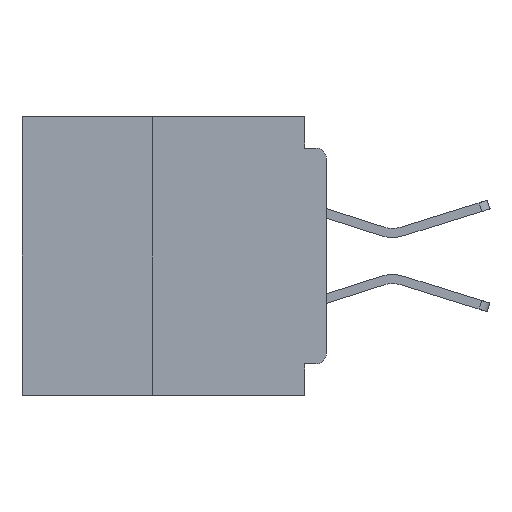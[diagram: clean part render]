
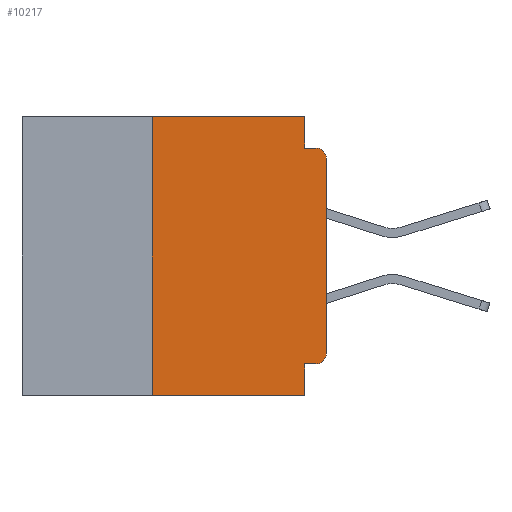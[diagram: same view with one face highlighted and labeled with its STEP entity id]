
A CAD part, left-side view. The second image highlights one B-rep face of the part: STEP entity #10217.
In plain terms, the highlighted planar face has unit normal (-1, 0, 0).
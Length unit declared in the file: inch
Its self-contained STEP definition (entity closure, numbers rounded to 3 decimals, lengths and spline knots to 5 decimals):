
#498 = CIRCLE ( 'NONE', #4912, 0.015 ) ;
#884 = EDGE_CURVE ( 'NONE', #46273, #10649, #34184, .T. ) ;
#911 = ORIENTED_EDGE ( 'NONE', *, *, #20412, .F. ) ;
#1662 = AXIS2_PLACEMENT_3D ( 'NONE', #39921, #15898, #43941 ) ;
#2048 = ORIENTED_EDGE ( 'NONE', *, *, #2463, .F. ) ;
#2142 = VERTEX_POINT ( 'NONE', #7467 ) ;
#2463 = EDGE_CURVE ( 'NONE', #22244, #46273, #28399, .T. ) ;
#3610 = EDGE_CURVE ( 'NONE', #47137, #48964, #48916, .T. ) ;
#3643 = ORIENTED_EDGE ( 'NONE', *, *, #884, .F. ) ;
#4256 = CARTESIAN_POINT ( 'NONE',  ( 0., 0., -0.045 ) ) ;
#4887 = DIRECTION ( 'NONE',  ( 0., -1., 0. ) ) ;
#4912 = AXIS2_PLACEMENT_3D ( 'NONE', #46731, #22721, #50726 ) ;
#5060 = CARTESIAN_POINT ( 'NONE',  ( 0., 0.031, 0. ) ) ;
#5087 = VECTOR ( 'NONE', #30559, 39.37008 ) ;
#5293 = CARTESIAN_POINT ( 'NONE',  ( 0., 0.031, 0. ) ) ;
#6750 = LINE ( 'NONE', #5293, #48163 ) ;
#7467 = CARTESIAN_POINT ( 'NONE',  ( 0., 0.031, -0.4 ) ) ;
#7532 = DIRECTION ( 'NONE',  ( 0., -1., 0. ) ) ;
#7819 = EDGE_CURVE ( 'NONE', #34280, #49689, #32407, .T. ) ;
#7886 = LINE ( 'NONE', #27596, #49278 ) ;
#9709 = DIRECTION ( 'NONE',  ( 0., 1., 0. ) ) ;
#10217 = ADVANCED_FACE ( 'NONE', ( #42195 ), #37605, .F. ) ;
#10649 = VERTEX_POINT ( 'NONE', #5060 ) ;
#10963 = EDGE_CURVE ( 'NONE', #33934, #2142, #45840, .T. ) ;
#11581 = CARTESIAN_POINT ( 'NONE',  ( 0., 0.25, -0.4 ) ) ;
#12179 = EDGE_LOOP ( 'NONE', ( #19804, #41175, #29316, #911, #3643, #2048, #46220, #25577, #29150, #15130 ) ) ;
#13607 = CARTESIAN_POINT ( 'NONE',  ( 0., 0.437, 0. ) ) ;
#13800 = CARTESIAN_POINT ( 'NONE',  ( 0., 0.25, 0. ) ) ;
#14956 = CARTESIAN_POINT ( 'NONE',  ( 0., 0.015, -0.355 ) ) ;
#15130 = ORIENTED_EDGE ( 'NONE', *, *, #7819, .T. ) ;
#15285 = DIRECTION ( 'NONE',  ( 0., 0., -1. ) ) ;
#15851 = LINE ( 'NONE', #50484, #5087 ) ;
#15898 = DIRECTION ( 'NONE',  ( -1., 0., 0. ) ) ;
#17641 = DIRECTION ( 'NONE',  ( 0., 0., -1. ) ) ;
#17723 = VECTOR ( 'NONE', #36551, 39.37008 ) ;
#19588 = VERTEX_POINT ( 'NONE', #20359 ) ;
#19804 = ORIENTED_EDGE ( 'NONE', *, *, #39265, .T. ) ;
#20359 = CARTESIAN_POINT ( 'NONE',  ( 0., 0., -0.06 ) ) ;
#20412 = EDGE_CURVE ( 'NONE', #10649, #47137, #6750, .T. ) ;
#22244 = VERTEX_POINT ( 'NONE', #11581 ) ;
#22721 = DIRECTION ( 'NONE',  ( -1., 0., 0. ) ) ;
#24811 = VECTOR ( 'NONE', #25197, 39.37008 ) ;
#25197 = DIRECTION ( 'NONE',  ( 0., -1., 0. ) ) ;
#25252 = CARTESIAN_POINT ( 'NONE',  ( 0., 0.437, 0. ) ) ;
#25577 = ORIENTED_EDGE ( 'NONE', *, *, #10963, .F. ) ;
#27596 = CARTESIAN_POINT ( 'NONE',  ( 0., 0.437, -0.4 ) ) ;
#27672 = VECTOR ( 'NONE', #4887, 39.37008 ) ;
#28399 = LINE ( 'NONE', #39073, #17723 ) ;
#28446 = EDGE_CURVE ( 'NONE', #34280, #33934, #32401, .T. ) ;
#28682 = CARTESIAN_POINT ( 'NONE',  ( 0., 0.031, -0.355 ) ) ;
#28780 = EDGE_CURVE ( 'NONE', #22244, #2142, #7886, .T. ) ;
#29150 = ORIENTED_EDGE ( 'NONE', *, *, #28446, .F. ) ;
#29316 = ORIENTED_EDGE ( 'NONE', *, *, #3610, .F. ) ;
#29700 = CARTESIAN_POINT ( 'NONE',  ( 0., 0., -0.355 ) ) ;
#30559 = DIRECTION ( 'NONE',  ( 0., 0., 1. ) ) ;
#32401 = LINE ( 'NONE', #29700, #41838 ) ;
#32407 = CIRCLE ( 'NONE', #1662, 0.015 ) ;
#33437 = CARTESIAN_POINT ( 'NONE',  ( 0., 0., -0.34 ) ) ;
#33934 = VERTEX_POINT ( 'NONE', #28682 ) ;
#34184 = LINE ( 'NONE', #25252, #24811 ) ;
#34280 = VERTEX_POINT ( 'NONE', #14956 ) ;
#34900 = CARTESIAN_POINT ( 'NONE',  ( 0., 0.031, -0.045 ) ) ;
#35152 = VECTOR ( 'NONE', #15285, 39.37008 ) ;
#36551 = DIRECTION ( 'NONE',  ( 0., 0., 1. ) ) ;
#37605 = PLANE ( 'NONE',  #51189 ) ;
#39073 = CARTESIAN_POINT ( 'NONE',  ( 0., 0.25, -0.4 ) ) ;
#39265 = EDGE_CURVE ( 'NONE', #49689, #19588, #15851, .T. ) ;
#39317 = CARTESIAN_POINT ( 'NONE',  ( 0., 0.031, -0.4 ) ) ;
#39921 = CARTESIAN_POINT ( 'NONE',  ( 0., 0.015, -0.34 ) ) ;
#40498 = EDGE_CURVE ( 'NONE', #19588, #48964, #498, .T. ) ;
#41175 = ORIENTED_EDGE ( 'NONE', *, *, #40498, .T. ) ;
#41501 = DIRECTION ( 'NONE',  ( 0., 0., -1. ) ) ;
#41660 = DIRECTION ( 'NONE',  ( 1., 0., 0. ) ) ;
#41838 = VECTOR ( 'NONE', #9709, 39.37008 ) ;
#42195 = FACE_OUTER_BOUND ( 'NONE', #12179, .T. ) ;
#43941 = DIRECTION ( 'NONE',  ( 0., 0., -1. ) ) ;
#44570 = CARTESIAN_POINT ( 'NONE',  ( 0., 0.015, -0.045 ) ) ;
#45840 = LINE ( 'NONE', #39317, #35152 ) ;
#46220 = ORIENTED_EDGE ( 'NONE', *, *, #28780, .T. ) ;
#46273 = VERTEX_POINT ( 'NONE', #13800 ) ;
#46731 = CARTESIAN_POINT ( 'NONE',  ( 0., 0.015, -0.06 ) ) ;
#47137 = VERTEX_POINT ( 'NONE', #34900 ) ;
#48163 = VECTOR ( 'NONE', #41501, 39.37008 ) ;
#48916 = LINE ( 'NONE', #4256, #27672 ) ;
#48964 = VERTEX_POINT ( 'NONE', #44570 ) ;
#49278 = VECTOR ( 'NONE', #7532, 39.37008 ) ;
#49689 = VERTEX_POINT ( 'NONE', #33437 ) ;
#50484 = CARTESIAN_POINT ( 'NONE',  ( 0., 0., 0. ) ) ;
#50726 = DIRECTION ( 'NONE',  ( 0., 0., -1. ) ) ;
#51189 = AXIS2_PLACEMENT_3D ( 'NONE', #13607, #41660, #17641 ) ;
